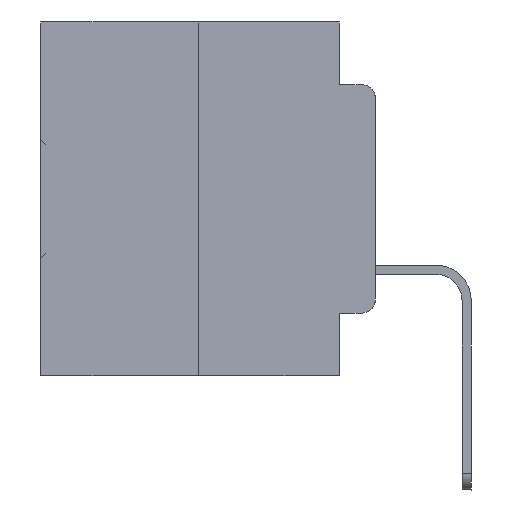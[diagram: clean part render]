
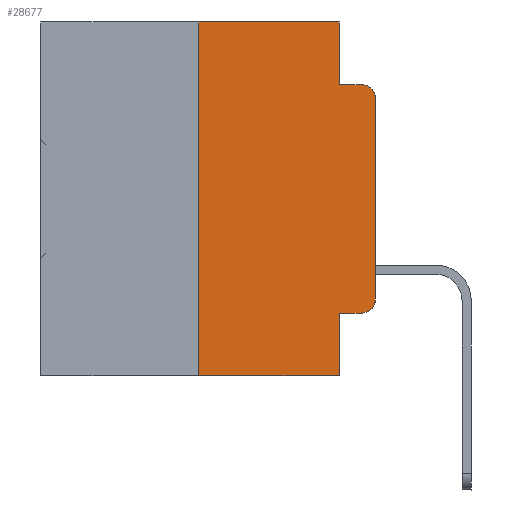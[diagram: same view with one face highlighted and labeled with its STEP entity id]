
A CAD part, left-side view. The second image highlights one B-rep face of the part: STEP entity #28677.
In plain terms, the highlighted planar face has unit normal (-1, 0, 0).
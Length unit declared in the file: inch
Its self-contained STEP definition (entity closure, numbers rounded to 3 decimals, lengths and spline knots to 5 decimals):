
#903 = DIRECTION ( 'NONE',  ( 0., 0., -1. ) ) ;
#909 = VECTOR ( 'NONE', #29695, 39.37008 ) ;
#1126 = EDGE_CURVE ( 'NONE', #27273, #25673, #24289, .T. ) ;
#1542 = ORIENTED_EDGE ( 'NONE', *, *, #16643, .T. ) ;
#1778 = CARTESIAN_POINT ( 'NONE',  ( 0., 0.473, -0.5 ) ) ;
#2188 = CARTESIAN_POINT ( 'NONE',  ( 0., 0.25, 0. ) ) ;
#2589 = CARTESIAN_POINT ( 'NONE',  ( 0., 0.02, -0.1085 ) ) ;
#2701 = DIRECTION ( 'NONE',  ( -1., 0., 0. ) ) ;
#2780 = VERTEX_POINT ( 'NONE', #30583 ) ;
#3193 = AXIS2_PLACEMENT_3D ( 'NONE', #2589, #2701, #18256 ) ;
#3331 = CIRCLE ( 'NONE', #3193, 0.02 ) ;
#3581 = DIRECTION ( 'NONE',  ( 0., -1., 0. ) ) ;
#3712 = ORIENTED_EDGE ( 'NONE', *, *, #27208, .T. ) ;
#3947 = VECTOR ( 'NONE', #10344, 39.37008 ) ;
#4598 = ORIENTED_EDGE ( 'NONE', *, *, #20807, .T. ) ;
#5251 = LINE ( 'NONE', #1778, #31664 ) ;
#5803 = EDGE_CURVE ( 'NONE', #24756, #9394, #24395, .T. ) ;
#5935 = LINE ( 'NONE', #16449, #19559 ) ;
#6324 = EDGE_CURVE ( 'NONE', #9394, #27273, #5935, .T. ) ;
#7860 = ORIENTED_EDGE ( 'NONE', *, *, #13061, .T. ) ;
#7936 = CARTESIAN_POINT ( 'NONE',  ( 0., 0.051, -0.5 ) ) ;
#8819 = EDGE_CURVE ( 'NONE', #25066, #25558, #19763, .T. ) ;
#9394 = VERTEX_POINT ( 'NONE', #11542 ) ;
#10344 = DIRECTION ( 'NONE',  ( 0., -1., 0. ) ) ;
#10662 = VECTOR ( 'NONE', #28843, 39.37008 ) ;
#11373 = ORIENTED_EDGE ( 'NONE', *, *, #8819, .F. ) ;
#11542 = CARTESIAN_POINT ( 'NONE',  ( 0., 0.25, 0. ) ) ;
#11602 = CARTESIAN_POINT ( 'NONE',  ( 0., 0.051, -0.4115 ) ) ;
#12044 = DIRECTION ( 'NONE',  ( 0., -1., 0. ) ) ;
#12800 = CARTESIAN_POINT ( 'NONE',  ( 0., 0.051, -0.0885 ) ) ;
#13061 = EDGE_CURVE ( 'NONE', #27785, #18146, #13798, .T. ) ;
#13413 = CARTESIAN_POINT ( 'NONE',  ( 0., 0.051, -0.0885 ) ) ;
#13798 = CIRCLE ( 'NONE', #21355, 0.02 ) ;
#13918 = CARTESIAN_POINT ( 'NONE',  ( 0., 0.02, -0.4115 ) ) ;
#14105 = EDGE_CURVE ( 'NONE', #25673, #2780, #18369, .T. ) ;
#14269 = CARTESIAN_POINT ( 'NONE',  ( 0., 0.25, -0.5 ) ) ;
#14354 = CARTESIAN_POINT ( 'NONE',  ( 0., 0., -0.1085 ) ) ;
#15101 = DIRECTION ( 'NONE',  ( 0., 0., -1. ) ) ;
#15295 = ORIENTED_EDGE ( 'NONE', *, *, #14105, .F. ) ;
#16449 = CARTESIAN_POINT ( 'NONE',  ( 0., 0.473, 0. ) ) ;
#16643 = EDGE_CURVE ( 'NONE', #20318, #2780, #3331, .T. ) ;
#16667 = ORIENTED_EDGE ( 'NONE', *, *, #26045, .T. ) ;
#16726 = VECTOR ( 'NONE', #24621, 39.37008 ) ;
#18146 = VERTEX_POINT ( 'NONE', #30751 ) ;
#18256 = DIRECTION ( 'NONE',  ( 0., 0., -1. ) ) ;
#18369 = LINE ( 'NONE', #12800, #3947 ) ;
#18536 = AXIS2_PLACEMENT_3D ( 'NONE', #30449, #32671, #15101 ) ;
#19559 = VECTOR ( 'NONE', #3581, 39.37008 ) ;
#19589 = CARTESIAN_POINT ( 'NONE',  ( 0., 0.051, 0. ) ) ;
#19728 = EDGE_LOOP ( 'NONE', ( #4598, #1542, #15295, #29970, #26211, #26454, #16667, #11373, #3712, #7860 ) ) ;
#19763 = LINE ( 'NONE', #27460, #909 ) ;
#20017 = VECTOR ( 'NONE', #27816, 39.37008 ) ;
#20318 = VERTEX_POINT ( 'NONE', #14354 ) ;
#20807 = EDGE_CURVE ( 'NONE', #18146, #20318, #23168, .T. ) ;
#21355 = AXIS2_PLACEMENT_3D ( 'NONE', #28894, #31576, #903 ) ;
#23168 = LINE ( 'NONE', #24261, #31958 ) ;
#23490 = CARTESIAN_POINT ( 'NONE',  ( 0., 0.051, 0. ) ) ;
#23508 = FACE_OUTER_BOUND ( 'NONE', #19728, .T. ) ;
#24261 = CARTESIAN_POINT ( 'NONE',  ( 0., 0., 0. ) ) ;
#24289 = LINE ( 'NONE', #23490, #10662 ) ;
#24395 = LINE ( 'NONE', #2188, #20017 ) ;
#24621 = DIRECTION ( 'NONE',  ( 0., -1., 0. ) ) ;
#24756 = VERTEX_POINT ( 'NONE', #14269 ) ;
#25066 = VERTEX_POINT ( 'NONE', #31483 ) ;
#25558 = VERTEX_POINT ( 'NONE', #7936 ) ;
#25673 = VERTEX_POINT ( 'NONE', #13413 ) ;
#26045 = EDGE_CURVE ( 'NONE', #24756, #25558, #5251, .T. ) ;
#26211 = ORIENTED_EDGE ( 'NONE', *, *, #6324, .F. ) ;
#26454 = ORIENTED_EDGE ( 'NONE', *, *, #5803, .F. ) ;
#27208 = EDGE_CURVE ( 'NONE', #25066, #27785, #29543, .T. ) ;
#27273 = VERTEX_POINT ( 'NONE', #19589 ) ;
#27460 = CARTESIAN_POINT ( 'NONE',  ( 0., 0.051, 0. ) ) ;
#27644 = PLANE ( 'NONE',  #18536 ) ;
#27785 = VERTEX_POINT ( 'NONE', #13918 ) ;
#27816 = DIRECTION ( 'NONE',  ( 0., 0., 1. ) ) ;
#28677 = ADVANCED_FACE ( 'NONE', ( #23508 ), #27644, .F. ) ;
#28843 = DIRECTION ( 'NONE',  ( 0., 0., -1. ) ) ;
#28894 = CARTESIAN_POINT ( 'NONE',  ( 0., 0.02, -0.3915 ) ) ;
#29293 = DIRECTION ( 'NONE',  ( 0., 0., 1. ) ) ;
#29543 = LINE ( 'NONE', #11602, #16726 ) ;
#29695 = DIRECTION ( 'NONE',  ( 0., 0., -1. ) ) ;
#29970 = ORIENTED_EDGE ( 'NONE', *, *, #1126, .F. ) ;
#30449 = CARTESIAN_POINT ( 'NONE',  ( 0., 0.473, 0. ) ) ;
#30583 = CARTESIAN_POINT ( 'NONE',  ( 0., 0.02, -0.0885 ) ) ;
#30751 = CARTESIAN_POINT ( 'NONE',  ( 0., 0., -0.3915 ) ) ;
#31483 = CARTESIAN_POINT ( 'NONE',  ( 0., 0.051, -0.4115 ) ) ;
#31576 = DIRECTION ( 'NONE',  ( -1., 0., 0. ) ) ;
#31664 = VECTOR ( 'NONE', #12044, 39.37008 ) ;
#31958 = VECTOR ( 'NONE', #29293, 39.37008 ) ;
#32671 = DIRECTION ( 'NONE',  ( 1., 0., 0. ) ) ;
